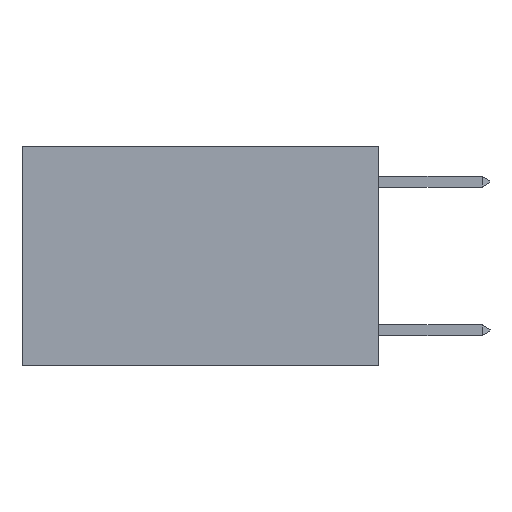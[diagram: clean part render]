
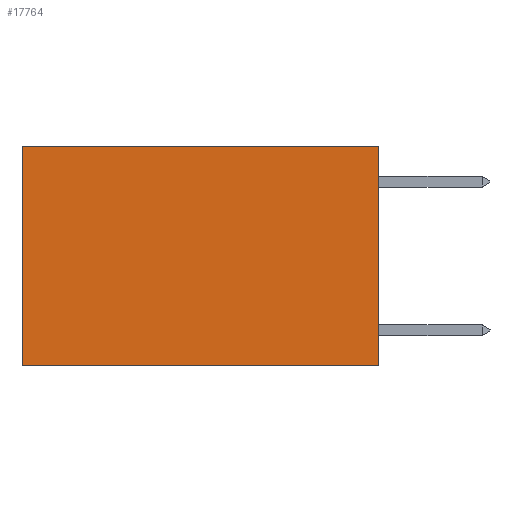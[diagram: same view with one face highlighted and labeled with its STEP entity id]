
A CAD part, left-side view. The second image highlights one B-rep face of the part: STEP entity #17764.
In plain terms, the highlighted planar face has unit normal (-1, 0, 0).
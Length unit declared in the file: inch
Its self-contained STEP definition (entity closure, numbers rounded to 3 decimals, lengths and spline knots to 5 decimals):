
#173 = ORIENTED_EDGE ( 'NONE', *, *, #19617, .F. ) ;
#480 = EDGE_CURVE ( 'NONE', #24963, #2572, #18936, .T. ) ;
#773 = ORIENTED_EDGE ( 'NONE', *, *, #9125, .F. ) ;
#808 = EDGE_LOOP ( 'NONE', ( #14711, #173, #773, #16027 ) ) ;
#1792 = CARTESIAN_POINT ( 'NONE',  ( 0.2625, 0., 0. ) ) ;
#2372 = VECTOR ( 'NONE', #18899, 39.37008 ) ;
#2572 = VERTEX_POINT ( 'NONE', #8850 ) ;
#2925 = LINE ( 'NONE', #1792, #2372 ) ;
#4218 = FACE_OUTER_BOUND ( 'NONE', #808, .T. ) ;
#7977 = VERTEX_POINT ( 'NONE', #15246 ) ;
#8080 = DIRECTION ( 'NONE',  ( 0., 0., -1. ) ) ;
#8850 = CARTESIAN_POINT ( 'NONE',  ( 0.2625, 0.6, -0.37 ) ) ;
#8925 = LINE ( 'NONE', #20994, #19200 ) ;
#9125 = EDGE_CURVE ( 'NONE', #7977, #22158, #2925, .T. ) ;
#9172 = CARTESIAN_POINT ( 'NONE',  ( 0.2625, 0., -0.37 ) ) ;
#9879 = DIRECTION ( 'NONE',  ( 1., 0., 0. ) ) ;
#10724 = DIRECTION ( 'NONE',  ( 0., 1., 0. ) ) ;
#11874 = PLANE ( 'NONE',  #18028 ) ;
#12777 = CARTESIAN_POINT ( 'NONE',  ( 0.2625, 0., 0. ) ) ;
#14711 = ORIENTED_EDGE ( 'NONE', *, *, #480, .T. ) ;
#15246 = CARTESIAN_POINT ( 'NONE',  ( 0.2625, 0., 0. ) ) ;
#16027 = ORIENTED_EDGE ( 'NONE', *, *, #19607, .T. ) ;
#17764 = ADVANCED_FACE ( 'NONE', ( #4218 ), #11874, .F. ) ;
#18028 = AXIS2_PLACEMENT_3D ( 'NONE', #22083, #9879, #23986 ) ;
#18899 = DIRECTION ( 'NONE',  ( 0., 0., -1. ) ) ;
#18933 = VECTOR ( 'NONE', #8080, 39.37008 ) ;
#18936 = LINE ( 'NONE', #21281, #18933 ) ;
#19200 = VECTOR ( 'NONE', #22920, 39.37008 ) ;
#19607 = EDGE_CURVE ( 'NONE', #7977, #24963, #19844, .T. ) ;
#19617 = EDGE_CURVE ( 'NONE', #22158, #2572, #8925, .T. ) ;
#19844 = LINE ( 'NONE', #12777, #25608 ) ;
#20994 = CARTESIAN_POINT ( 'NONE',  ( 0.2625, 0., -0.37 ) ) ;
#21281 = CARTESIAN_POINT ( 'NONE',  ( 0.2625, 0.6, 0. ) ) ;
#22083 = CARTESIAN_POINT ( 'NONE',  ( 0.2625, 0., 0. ) ) ;
#22158 = VERTEX_POINT ( 'NONE', #9172 ) ;
#22920 = DIRECTION ( 'NONE',  ( 0., 1., 0. ) ) ;
#23919 = CARTESIAN_POINT ( 'NONE',  ( 0.2625, 0.6, 0. ) ) ;
#23986 = DIRECTION ( 'NONE',  ( 0., 0., -1. ) ) ;
#24963 = VERTEX_POINT ( 'NONE', #23919 ) ;
#25608 = VECTOR ( 'NONE', #10724, 39.37008 ) ;
